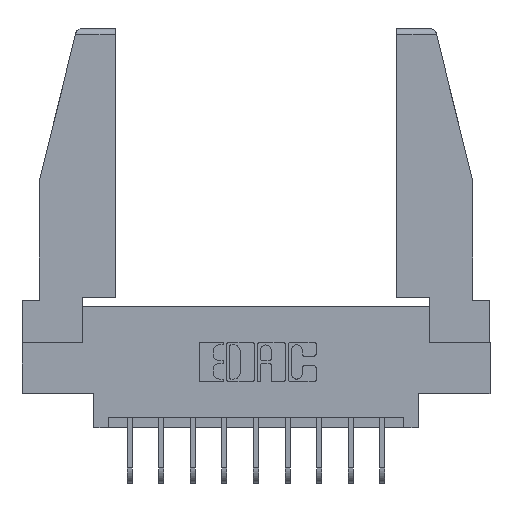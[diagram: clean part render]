
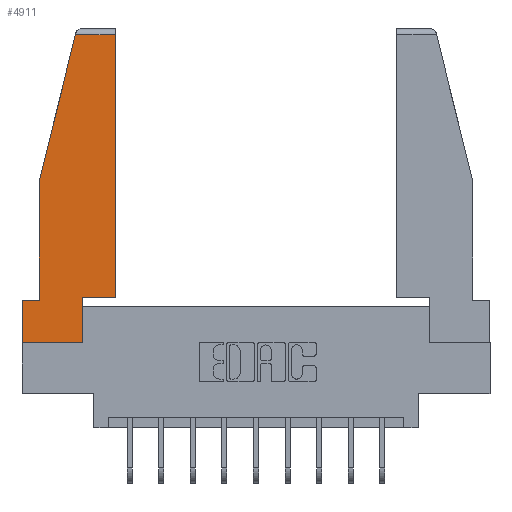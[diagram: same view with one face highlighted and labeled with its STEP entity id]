
A CAD part, top view. The second image highlights one B-rep face of the part: STEP entity #4911.
In plain terms, the highlighted planar face has unit normal (0, 0, 1).
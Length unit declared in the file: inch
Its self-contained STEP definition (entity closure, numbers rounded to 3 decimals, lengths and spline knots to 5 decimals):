
#259 = VECTOR ( 'NONE', #5290, 39.37008 ) ;
#328 = DIRECTION ( 'NONE',  ( 0., -1., 0. ) ) ;
#464 = EDGE_LOOP ( 'NONE', ( #2511, #9337, #1556, #786, #8841, #8071, #6025, #9936, #4473 ) ) ;
#786 = ORIENTED_EDGE ( 'NONE', *, *, #6856, .T. ) ;
#842 = VECTOR ( 'NONE', #9121, 39.37008 ) ;
#881 = CARTESIAN_POINT ( 'NONE',  ( 0.461, 0.223, 0. ) ) ;
#916 = CARTESIAN_POINT ( 'NONE',  ( 0., 0., 0. ) ) ;
#946 = AXIS2_PLACEMENT_3D ( 'NONE', #2622, #1567, #11085 ) ;
#1119 = VERTEX_POINT ( 'NONE', #4418 ) ;
#1391 = VERTEX_POINT ( 'NONE', #10856 ) ;
#1556 = ORIENTED_EDGE ( 'NONE', *, *, #7195, .T. ) ;
#1567 = DIRECTION ( 'NONE',  ( 0., 0., 1. ) ) ;
#1729 = CARTESIAN_POINT ( 'NONE',  ( 0., 0.21, 0. ) ) ;
#1854 = VERTEX_POINT ( 'NONE', #881 ) ;
#1932 = VECTOR ( 'NONE', #7510, 39.37008 ) ;
#1949 = DIRECTION ( 'NONE',  ( 0., -1., 0. ) ) ;
#2002 = CARTESIAN_POINT ( 'NONE',  ( 0.297, 0.223, 0. ) ) ;
#2219 = VECTOR ( 'NONE', #13576, 39.37008 ) ;
#2235 = VERTEX_POINT ( 'NONE', #916 ) ;
#2376 = CARTESIAN_POINT ( 'NONE',  ( 0., 1.52, 0. ) ) ;
#2511 = ORIENTED_EDGE ( 'NONE', *, *, #13303, .T. ) ;
#2579 = PLANE ( 'NONE',  #946 ) ;
#2622 = CARTESIAN_POINT ( 'NONE',  ( 0., 0., 0. ) ) ;
#2894 = VERTEX_POINT ( 'NONE', #9976 ) ;
#3146 = DIRECTION ( 'NONE',  ( 1., 0., 0. ) ) ;
#3520 = CARTESIAN_POINT ( 'NONE',  ( 0.2636, 1.52, 0. ) ) ;
#3728 = LINE ( 'NONE', #13022, #11142 ) ;
#3862 = LINE ( 'NONE', #2002, #2219 ) ;
#4395 = CARTESIAN_POINT ( 'NONE',  ( 0.297, 0.223, 0. ) ) ;
#4418 = CARTESIAN_POINT ( 'NONE',  ( 0.297, 0., 0. ) ) ;
#4473 = ORIENTED_EDGE ( 'NONE', *, *, #6802, .T. ) ;
#4588 = EDGE_CURVE ( 'NONE', #6470, #2235, #3728, .T. ) ;
#4631 = VECTOR ( 'NONE', #3146, 39.37008 ) ;
#4634 = VERTEX_POINT ( 'NONE', #3520 ) ;
#4911 = ADVANCED_FACE ( 'NONE', ( #11820 ), #2579, .T. ) ;
#5092 = EDGE_CURVE ( 'NONE', #1119, #7689, #8206, .T. ) ;
#5290 = DIRECTION ( 'NONE',  ( 0., 1., 0. ) ) ;
#5762 = LINE ( 'NONE', #11750, #4631 ) ;
#5835 = LINE ( 'NONE', #6857, #842 ) ;
#6016 = LINE ( 'NONE', #11323, #8492 ) ;
#6025 = ORIENTED_EDGE ( 'NONE', *, *, #11676, .T. ) ;
#6193 = CARTESIAN_POINT ( 'NONE',  ( 0.086, 0.8, 0. ) ) ;
#6331 = VECTOR ( 'NONE', #1949, 39.37008 ) ;
#6342 = CARTESIAN_POINT ( 'NONE',  ( 0.086, 0.8, 0. ) ) ;
#6470 = VERTEX_POINT ( 'NONE', #1729 ) ;
#6502 = LINE ( 'NONE', #6193, #6331 ) ;
#6802 = EDGE_CURVE ( 'NONE', #7689, #1854, #3862, .T. ) ;
#6856 = EDGE_CURVE ( 'NONE', #11082, #2894, #6502, .T. ) ;
#6857 = CARTESIAN_POINT ( 'NONE',  ( 0.271, 1.55, 0. ) ) ;
#6982 = EDGE_CURVE ( 'NONE', #1391, #4634, #9454, .T. ) ;
#7068 = CARTESIAN_POINT ( 'NONE',  ( 0.297, 0., 0. ) ) ;
#7195 = EDGE_CURVE ( 'NONE', #4634, #11082, #5835, .T. ) ;
#7498 = DIRECTION ( 'NONE',  ( -1., 0., 0. ) ) ;
#7510 = DIRECTION ( 'NONE',  ( 0., 1., 0. ) ) ;
#7689 = VERTEX_POINT ( 'NONE', #4395 ) ;
#8071 = ORIENTED_EDGE ( 'NONE', *, *, #4588, .T. ) ;
#8206 = LINE ( 'NONE', #7068, #259 ) ;
#8492 = VECTOR ( 'NONE', #10204, 39.37008 ) ;
#8841 = ORIENTED_EDGE ( 'NONE', *, *, #9041, .T. ) ;
#9041 = EDGE_CURVE ( 'NONE', #2894, #6470, #6016, .T. ) ;
#9119 = VECTOR ( 'NONE', #7498, 39.37008 ) ;
#9121 = DIRECTION ( 'NONE',  ( -0.239, -0.971, 0. ) ) ;
#9337 = ORIENTED_EDGE ( 'NONE', *, *, #6982, .T. ) ;
#9454 = LINE ( 'NONE', #2376, #9119 ) ;
#9936 = ORIENTED_EDGE ( 'NONE', *, *, #5092, .T. ) ;
#9976 = CARTESIAN_POINT ( 'NONE',  ( 0.086, 0.21, 0. ) ) ;
#10204 = DIRECTION ( 'NONE',  ( -1., 0., 0. ) ) ;
#10226 = CARTESIAN_POINT ( 'NONE',  ( 0.461, 0.223, 0. ) ) ;
#10856 = CARTESIAN_POINT ( 'NONE',  ( 0.461, 1.52, 0. ) ) ;
#11082 = VERTEX_POINT ( 'NONE', #6342 ) ;
#11085 = DIRECTION ( 'NONE',  ( 1., 0., 0. ) ) ;
#11142 = VECTOR ( 'NONE', #328, 39.37008 ) ;
#11323 = CARTESIAN_POINT ( 'NONE',  ( 0., 0.21, 0. ) ) ;
#11676 = EDGE_CURVE ( 'NONE', #2235, #1119, #5762, .T. ) ;
#11750 = CARTESIAN_POINT ( 'NONE',  ( 0., 0., 0. ) ) ;
#11820 = FACE_OUTER_BOUND ( 'NONE', #464, .T. ) ;
#13022 = CARTESIAN_POINT ( 'NONE',  ( 0., 0.21, 0. ) ) ;
#13303 = EDGE_CURVE ( 'NONE', #1854, #1391, #13442, .T. ) ;
#13442 = LINE ( 'NONE', #10226, #1932 ) ;
#13576 = DIRECTION ( 'NONE',  ( 1., 0., 0. ) ) ;
